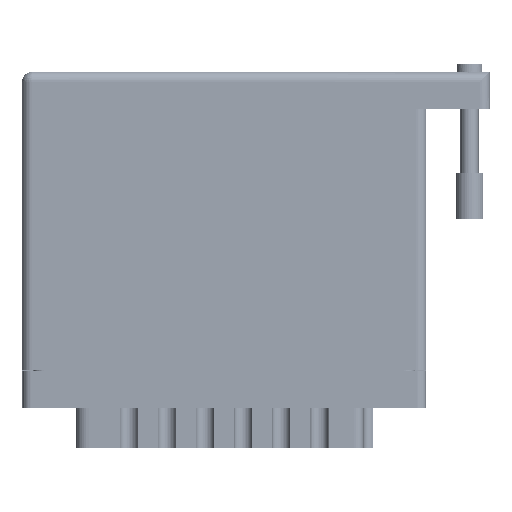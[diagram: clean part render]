
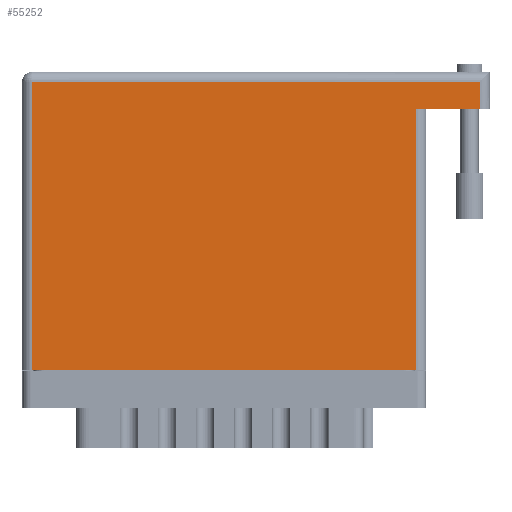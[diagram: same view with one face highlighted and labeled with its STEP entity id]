
A CAD part, front view. The second image highlights one B-rep face of the part: STEP entity #55252.
In plain terms, the highlighted face is planar.
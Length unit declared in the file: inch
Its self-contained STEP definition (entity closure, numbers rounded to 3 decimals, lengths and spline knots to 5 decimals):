
#329 = LINE ( 'NONE', #43527, #17164 ) ;
#2870 = DIRECTION ( 'NONE',  ( 0., 1., 0. ) ) ;
#4317 = VERTEX_POINT ( 'NONE', #77623 ) ;
#4762 = VERTEX_POINT ( 'NONE', #90238 ) ;
#6441 = DIRECTION ( 'NONE',  ( 0., 1., 0. ) ) ;
#9085 = DIRECTION ( 'NONE',  ( 1., 0., 0. ) ) ;
#10431 = VECTOR ( 'NONE', #79218, 39.37008 ) ;
#17164 = VECTOR ( 'NONE', #35996, 39.37008 ) ;
#19218 = AXIS2_PLACEMENT_3D ( 'NONE', #63266, #77379, #40735 ) ;
#19899 = ORIENTED_EDGE ( 'NONE', *, *, #28540, .T. ) ;
#20051 = FACE_OUTER_BOUND ( 'NONE', #63744, .T. ) ;
#21944 = VERTEX_POINT ( 'NONE', #83780 ) ;
#23956 = EDGE_CURVE ( 'NONE', #4317, #88427, #52175, .T. ) ;
#26429 = DIRECTION ( 'NONE',  ( -1., 0., 0. ) ) ;
#27300 = ORIENTED_EDGE ( 'NONE', *, *, #82871, .T. ) ;
#27597 = VECTOR ( 'NONE', #2870, 39.37008 ) ;
#28540 = EDGE_CURVE ( 'NONE', #21944, #4762, #64988, .T. ) ;
#29194 = VERTEX_POINT ( 'NONE', #91916 ) ;
#29220 = ORIENTED_EDGE ( 'NONE', *, *, #23956, .T. ) ;
#29908 = CARTESIAN_POINT ( 'NONE',  ( 0.07, 0., 0. ) ) ;
#32576 = CARTESIAN_POINT ( 'NONE',  ( 3.19, 1.774, 0. ) ) ;
#34792 = ORIENTED_EDGE ( 'NONE', *, *, #68454, .T. ) ;
#35996 = DIRECTION ( 'NONE',  ( -1., 0., 0. ) ) ;
#38548 = CARTESIAN_POINT ( 'NONE',  ( 3.12, 2.03, 0. ) ) ;
#40735 = DIRECTION ( 'NONE',  ( -1., 0., 0. ) ) ;
#41210 = LINE ( 'NONE', #42124, #88251 ) ;
#42124 = CARTESIAN_POINT ( 'NONE',  ( 2.685, 1.774, 0. ) ) ;
#43527 = CARTESIAN_POINT ( 'NONE',  ( 0., 1.96, 0. ) ) ;
#43844 = CARTESIAN_POINT ( 'NONE',  ( 0., 0., 0. ) ) ;
#45374 = EDGE_CURVE ( 'NONE', #4317, #79176, #90806, .T. ) ;
#52175 = LINE ( 'NONE', #38548, #27597 ) ;
#55252 = ADVANCED_FACE ( 'NONE', ( #20051 ), #83936, .F. ) ;
#55336 = EDGE_CURVE ( 'NONE', #4762, #79176, #41210, .T. ) ;
#62728 = ORIENTED_EDGE ( 'NONE', *, *, #55336, .T. ) ;
#63266 = CARTESIAN_POINT ( 'NONE',  ( 0., 2.03, 0. ) ) ;
#63744 = EDGE_LOOP ( 'NONE', ( #19899, #62728, #86973, #29220, #27300, #34792 ) ) ;
#64988 = LINE ( 'NONE', #43844, #91021 ) ;
#65163 = LINE ( 'NONE', #29908, #10431 ) ;
#68454 = EDGE_CURVE ( 'NONE', #29194, #21944, #65163, .T. ) ;
#70692 = VECTOR ( 'NONE', #26429, 39.37008 ) ;
#77379 = DIRECTION ( 'NONE',  ( 0., 0., -1. ) ) ;
#77623 = CARTESIAN_POINT ( 'NONE',  ( 3.12, 1.774, 0. ) ) ;
#79176 = VERTEX_POINT ( 'NONE', #83245 ) ;
#79218 = DIRECTION ( 'NONE',  ( 0., -1., 0. ) ) ;
#82871 = EDGE_CURVE ( 'NONE', #88427, #29194, #329, .T. ) ;
#83245 = CARTESIAN_POINT ( 'NONE',  ( 2.685, 1.774, 0. ) ) ;
#83780 = CARTESIAN_POINT ( 'NONE',  ( 0.07, 0., 0. ) ) ;
#83936 = PLANE ( 'NONE',  #19218 ) ;
#86973 = ORIENTED_EDGE ( 'NONE', *, *, #45374, .F. ) ;
#88111 = CARTESIAN_POINT ( 'NONE',  ( 3.12, 1.96, 0. ) ) ;
#88251 = VECTOR ( 'NONE', #6441, 39.37008 ) ;
#88427 = VERTEX_POINT ( 'NONE', #88111 ) ;
#90238 = CARTESIAN_POINT ( 'NONE',  ( 2.685, 0., 0. ) ) ;
#90806 = LINE ( 'NONE', #32576, #70692 ) ;
#91021 = VECTOR ( 'NONE', #9085, 39.37008 ) ;
#91916 = CARTESIAN_POINT ( 'NONE',  ( 0.07, 1.96, 0. ) ) ;
